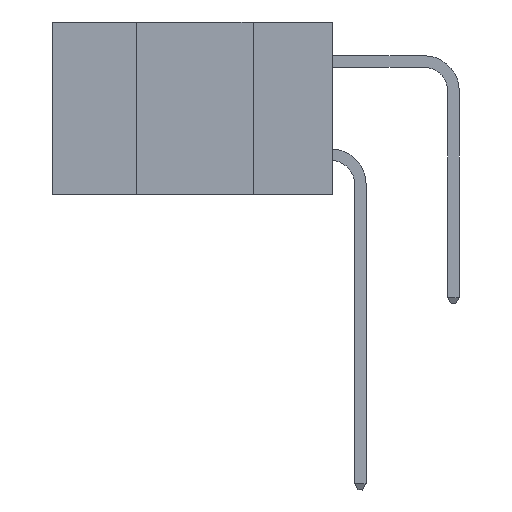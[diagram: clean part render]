
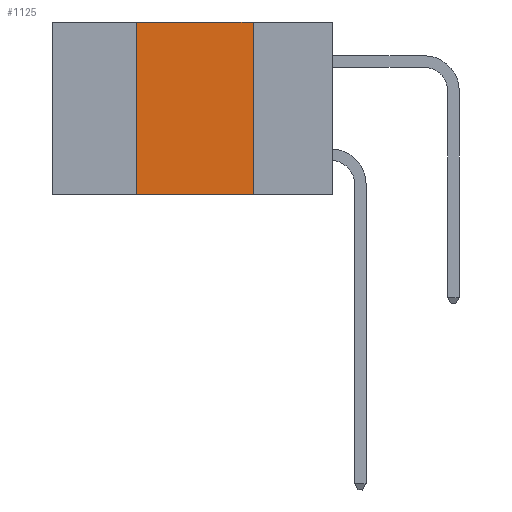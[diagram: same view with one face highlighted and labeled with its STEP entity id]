
A CAD part, left-side view. The second image highlights one B-rep face of the part: STEP entity #1125.
In plain terms, the highlighted planar face has unit normal (-1, 0, 0).
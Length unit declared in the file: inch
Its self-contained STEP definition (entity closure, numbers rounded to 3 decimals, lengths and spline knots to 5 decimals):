
#335 = DIRECTION ( 'NONE',  ( 0., 0., -1. ) ) ;
#376 = CARTESIAN_POINT ( 'NONE',  ( 0., 0.6, 0. ) ) ;
#490 = ORIENTED_EDGE ( 'NONE', *, *, #15571, .F. ) ;
#587 = DIRECTION ( 'NONE',  ( 1., 0., 0. ) ) ;
#1125 = ADVANCED_FACE ( 'NONE', ( #6624 ), #11788, .F. ) ;
#2198 = VECTOR ( 'NONE', #14328, 39.37008 ) ;
#2705 = ORIENTED_EDGE ( 'NONE', *, *, #8820, .F. ) ;
#4150 = VECTOR ( 'NONE', #9275, 39.37008 ) ;
#4286 = EDGE_CURVE ( 'NONE', #8039, #12441, #9489, .T. ) ;
#4405 = CARTESIAN_POINT ( 'NONE',  ( 0., 0.6, -0.37 ) ) ;
#4763 = CARTESIAN_POINT ( 'NONE',  ( 0., 0.42, -0.37 ) ) ;
#6476 = CARTESIAN_POINT ( 'NONE',  ( 0., 0.17, -0.37 ) ) ;
#6624 = FACE_OUTER_BOUND ( 'NONE', #10754, .T. ) ;
#7827 = EDGE_CURVE ( 'NONE', #15720, #13673, #9449, .T. ) ;
#7954 = VECTOR ( 'NONE', #8827, 39.37008 ) ;
#8039 = VERTEX_POINT ( 'NONE', #11307 ) ;
#8820 = EDGE_CURVE ( 'NONE', #13673, #12441, #16671, .T. ) ;
#8827 = DIRECTION ( 'NONE',  ( 0., 0., -1. ) ) ;
#9275 = DIRECTION ( 'NONE',  ( 0., -1., 0. ) ) ;
#9449 = LINE ( 'NONE', #376, #4150 ) ;
#9489 = LINE ( 'NONE', #4405, #2198 ) ;
#10081 = CARTESIAN_POINT ( 'NONE',  ( 0., 0.17, -0.37 ) ) ;
#10225 = AXIS2_PLACEMENT_3D ( 'NONE', #10519, #587, #335 ) ;
#10306 = CARTESIAN_POINT ( 'NONE',  ( 0., 0.17, 0. ) ) ;
#10519 = CARTESIAN_POINT ( 'NONE',  ( 0., 0.6, 0. ) ) ;
#10754 = EDGE_LOOP ( 'NONE', ( #2705, #13341, #490, #15250 ) ) ;
#11307 = CARTESIAN_POINT ( 'NONE',  ( 0., 0.42, -0.37 ) ) ;
#11788 = PLANE ( 'NONE',  #10225 ) ;
#12441 = VERTEX_POINT ( 'NONE', #10081 ) ;
#12980 = CARTESIAN_POINT ( 'NONE',  ( 0., 0.42, 0. ) ) ;
#13341 = ORIENTED_EDGE ( 'NONE', *, *, #7827, .F. ) ;
#13673 = VERTEX_POINT ( 'NONE', #10306 ) ;
#14034 = VECTOR ( 'NONE', #16653, 39.37008 ) ;
#14328 = DIRECTION ( 'NONE',  ( 0., -1., 0. ) ) ;
#15250 = ORIENTED_EDGE ( 'NONE', *, *, #4286, .T. ) ;
#15365 = LINE ( 'NONE', #4763, #14034 ) ;
#15571 = EDGE_CURVE ( 'NONE', #8039, #15720, #15365, .T. ) ;
#15720 = VERTEX_POINT ( 'NONE', #12980 ) ;
#16653 = DIRECTION ( 'NONE',  ( 0., 0., 1. ) ) ;
#16671 = LINE ( 'NONE', #6476, #7954 ) ;
